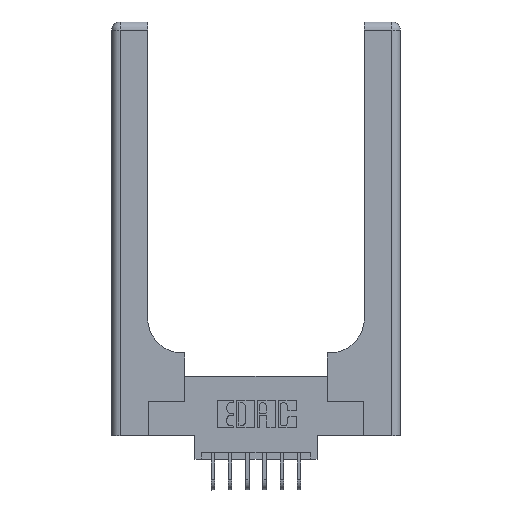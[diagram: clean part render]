
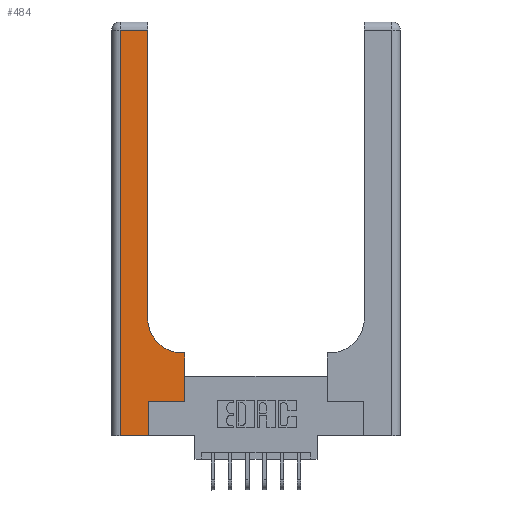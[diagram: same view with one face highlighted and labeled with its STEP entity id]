
A CAD part, top view. The second image highlights one B-rep face of the part: STEP entity #484.
In plain terms, the highlighted planar face has unit normal (0, 0, 1).
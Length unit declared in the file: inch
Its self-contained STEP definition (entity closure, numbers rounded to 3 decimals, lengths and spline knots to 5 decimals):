
#293 = EDGE_CURVE ( 'NONE', #11181, #2621, #364, .T. ) ;
#364 = LINE ( 'NONE', #6152, #12483 ) ;
#484 = ADVANCED_FACE ( 'NONE', ( #11495 ), #3996, .F. ) ;
#926 = DIRECTION ( 'NONE',  ( -1., 0., 0. ) ) ;
#940 = CARTESIAN_POINT ( 'NONE',  ( 0.51, 0.85, 0.37 ) ) ;
#962 = LINE ( 'NONE', #5746, #3664 ) ;
#1115 = DIRECTION ( 'NONE',  ( 0., 1., 0. ) ) ;
#1190 = ORIENTED_EDGE ( 'NONE', *, *, #2432, .T. ) ;
#1375 = CARTESIAN_POINT ( 'NONE',  ( 0.528, 0.25, 0.37 ) ) ;
#1651 = VERTEX_POINT ( 'NONE', #2572 ) ;
#1691 = VERTEX_POINT ( 'NONE', #7582 ) ;
#1703 = VECTOR ( 'NONE', #10372, 39.37008 ) ;
#2275 = VECTOR ( 'NONE', #6812, 39.37008 ) ;
#2432 = EDGE_CURVE ( 'NONE', #3363, #12640, #8522, .T. ) ;
#2565 = VERTEX_POINT ( 'NONE', #12368 ) ;
#2572 = CARTESIAN_POINT ( 'NONE',  ( 0.06, 0., 0.37 ) ) ;
#2621 = VERTEX_POINT ( 'NONE', #1375 ) ;
#2776 = EDGE_CURVE ( 'NONE', #6579, #1691, #5553, .T. ) ;
#2946 = CARTESIAN_POINT ( 'NONE',  ( 0., 0., 0.37 ) ) ;
#2987 = DIRECTION ( 'NONE',  ( 0., 0., -1. ) ) ;
#3363 = VERTEX_POINT ( 'NONE', #4736 ) ;
#3664 = VECTOR ( 'NONE', #926, 39.37008 ) ;
#3996 = PLANE ( 'NONE',  #13746 ) ;
#4009 = EDGE_CURVE ( 'NONE', #12640, #2565, #962, .T. ) ;
#4404 = EDGE_CURVE ( 'NONE', #2565, #1651, #7887, .T. ) ;
#4588 = CARTESIAN_POINT ( 'NONE',  ( 0.265, 0., 0.37 ) ) ;
#4621 = VECTOR ( 'NONE', #12848, 39.37008 ) ;
#4736 = CARTESIAN_POINT ( 'NONE',  ( 0.26, 0.85, 0.37 ) ) ;
#5387 = ORIENTED_EDGE ( 'NONE', *, *, #12440, .T. ) ;
#5443 = LINE ( 'NONE', #4588, #14311 ) ;
#5553 = LINE ( 'NONE', #15542, #2275 ) ;
#5615 = DIRECTION ( 'NONE',  ( -1., 0., 0. ) ) ;
#5627 = CARTESIAN_POINT ( 'NONE',  ( 0.06, 3., 0.37 ) ) ;
#5715 = CARTESIAN_POINT ( 'NONE',  ( 0.26, 3., 0.37 ) ) ;
#5742 = EDGE_LOOP ( 'NONE', ( #1190, #8745, #13155, #12164, #5387, #7445, #9410, #14818, #12945 ) ) ;
#5746 = CARTESIAN_POINT ( 'NONE',  ( 0., 2.94, 0.37 ) ) ;
#5777 = DIRECTION ( 'NONE',  ( 0., -1., 0. ) ) ;
#6152 = CARTESIAN_POINT ( 'NONE',  ( 0.265, 0.25, 0.37 ) ) ;
#6412 = CARTESIAN_POINT ( 'NONE',  ( 0.528, 0.25, 0.37 ) ) ;
#6579 = VERTEX_POINT ( 'NONE', #12979 ) ;
#6812 = DIRECTION ( 'NONE',  ( -1., 0., 0. ) ) ;
#7445 = ORIENTED_EDGE ( 'NONE', *, *, #293, .T. ) ;
#7582 = CARTESIAN_POINT ( 'NONE',  ( 0.51, 0.6, 0.37 ) ) ;
#7887 = LINE ( 'NONE', #5627, #15711 ) ;
#7896 = CARTESIAN_POINT ( 'NONE',  ( 0.26, 2.94, 0.37 ) ) ;
#8125 = VECTOR ( 'NONE', #1115, 39.37008 ) ;
#8244 = EDGE_CURVE ( 'NONE', #1651, #9885, #10815, .T. ) ;
#8522 = LINE ( 'NONE', #5715, #8125 ) ;
#8745 = ORIENTED_EDGE ( 'NONE', *, *, #4009, .T. ) ;
#9410 = ORIENTED_EDGE ( 'NONE', *, *, #15238, .T. ) ;
#9664 = CARTESIAN_POINT ( 'NONE',  ( 0.265, 0.25, 0.37 ) ) ;
#9698 = DIRECTION ( 'NONE',  ( 0., 0., -1. ) ) ;
#9746 = CARTESIAN_POINT ( 'NONE',  ( 0.265, 0., 0.37 ) ) ;
#9885 = VERTEX_POINT ( 'NONE', #9746 ) ;
#10372 = DIRECTION ( 'NONE',  ( 0., 1., 0. ) ) ;
#10460 = CARTESIAN_POINT ( 'NONE',  ( 0., 3., 0.37 ) ) ;
#10658 = EDGE_CURVE ( 'NONE', #1691, #3363, #14827, .T. ) ;
#10815 = LINE ( 'NONE', #2946, #4621 ) ;
#11145 = DIRECTION ( 'NONE',  ( 1., 0., 0. ) ) ;
#11181 = VERTEX_POINT ( 'NONE', #9664 ) ;
#11495 = FACE_OUTER_BOUND ( 'NONE', #5742, .T. ) ;
#12072 = AXIS2_PLACEMENT_3D ( 'NONE', #940, #9698, #14572 ) ;
#12164 = ORIENTED_EDGE ( 'NONE', *, *, #8244, .T. ) ;
#12368 = CARTESIAN_POINT ( 'NONE',  ( 0.06, 2.94, 0.37 ) ) ;
#12440 = EDGE_CURVE ( 'NONE', #9885, #11181, #5443, .T. ) ;
#12483 = VECTOR ( 'NONE', #11145, 39.37008 ) ;
#12640 = VERTEX_POINT ( 'NONE', #7896 ) ;
#12848 = DIRECTION ( 'NONE',  ( 1., 0., 0. ) ) ;
#12945 = ORIENTED_EDGE ( 'NONE', *, *, #10658, .T. ) ;
#12979 = CARTESIAN_POINT ( 'NONE',  ( 0.528, 0.6, 0.37 ) ) ;
#13155 = ORIENTED_EDGE ( 'NONE', *, *, #4404, .T. ) ;
#13299 = DIRECTION ( 'NONE',  ( 0., 1., 0. ) ) ;
#13641 = LINE ( 'NONE', #6412, #1703 ) ;
#13746 = AXIS2_PLACEMENT_3D ( 'NONE', #10460, #2987, #5615 ) ;
#14311 = VECTOR ( 'NONE', #13299, 39.37008 ) ;
#14572 = DIRECTION ( 'NONE',  ( 1., 0., 0. ) ) ;
#14818 = ORIENTED_EDGE ( 'NONE', *, *, #2776, .T. ) ;
#14827 = CIRCLE ( 'NONE', #12072, 0.25 ) ;
#15238 = EDGE_CURVE ( 'NONE', #2621, #6579, #13641, .T. ) ;
#15542 = CARTESIAN_POINT ( 'NONE',  ( 0.26, 0.6, 0.37 ) ) ;
#15711 = VECTOR ( 'NONE', #5777, 39.37008 ) ;
